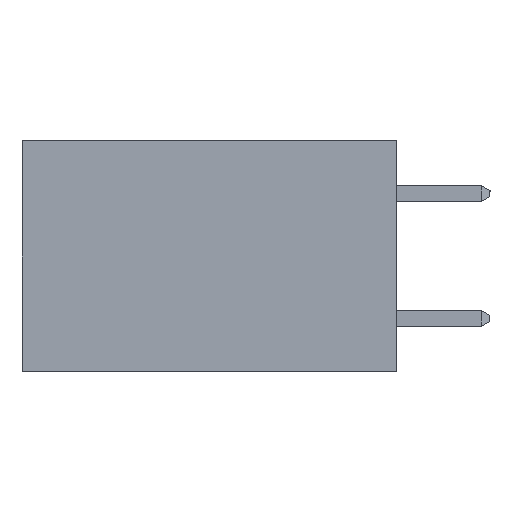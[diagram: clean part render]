
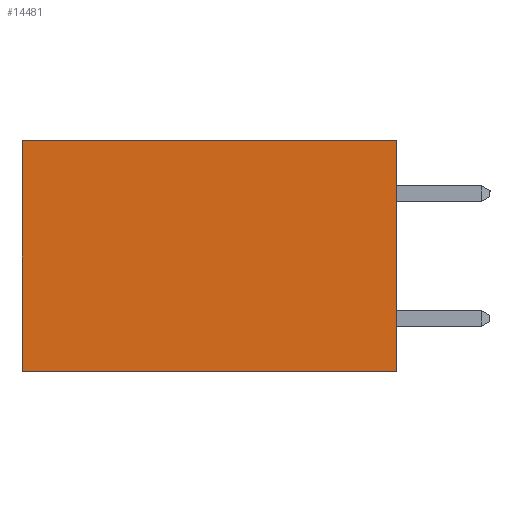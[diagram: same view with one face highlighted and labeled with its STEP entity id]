
A CAD part, left-side view. The second image highlights one B-rep face of the part: STEP entity #14481.
In plain terms, the highlighted planar face has unit normal (-1, 0, 0).
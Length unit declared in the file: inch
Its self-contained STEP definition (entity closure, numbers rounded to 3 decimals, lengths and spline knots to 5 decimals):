
#33 = VECTOR ( 'NONE', #13741, 39.37008 ) ;
#1514 = VECTOR ( 'NONE', #9625, 39.37008 ) ;
#1615 = VERTEX_POINT ( 'NONE', #4444 ) ;
#2081 = DIRECTION ( 'NONE',  ( 1., 0., 0. ) ) ;
#2562 = DIRECTION ( 'NONE',  ( 0., 0., -1. ) ) ;
#2619 = CARTESIAN_POINT ( 'NONE',  ( 0.2615, 0.6, 0. ) ) ;
#3501 = EDGE_CURVE ( 'NONE', #15536, #7044, #13768, .T. ) ;
#4334 = VECTOR ( 'NONE', #6171, 39.37008 ) ;
#4377 = CARTESIAN_POINT ( 'NONE',  ( 0.2615, 0., 0. ) ) ;
#4424 = CARTESIAN_POINT ( 'NONE',  ( 0.2615, 0., -0.37 ) ) ;
#4444 = CARTESIAN_POINT ( 'NONE',  ( 0.2615, 0., -0.37 ) ) ;
#4567 = ORIENTED_EDGE ( 'NONE', *, *, #15018, .F. ) ;
#5959 = LINE ( 'NONE', #11016, #4334 ) ;
#6171 = DIRECTION ( 'NONE',  ( 0., 1., 0. ) ) ;
#7044 = VERTEX_POINT ( 'NONE', #12034 ) ;
#7338 = AXIS2_PLACEMENT_3D ( 'NONE', #16398, #2081, #14927 ) ;
#7967 = ORIENTED_EDGE ( 'NONE', *, *, #3501, .T. ) ;
#8434 = EDGE_CURVE ( 'NONE', #1615, #7044, #5959, .T. ) ;
#9625 = DIRECTION ( 'NONE',  ( 0., 1., 0. ) ) ;
#11016 = CARTESIAN_POINT ( 'NONE',  ( 0.2615, 0., -0.37 ) ) ;
#11141 = ORIENTED_EDGE ( 'NONE', *, *, #14221, .T. ) ;
#11490 = EDGE_LOOP ( 'NONE', ( #7967, #15011, #4567, #11141 ) ) ;
#12034 = CARTESIAN_POINT ( 'NONE',  ( 0.2615, 0.6, -0.37 ) ) ;
#13741 = DIRECTION ( 'NONE',  ( 0., 0., -1. ) ) ;
#13768 = LINE ( 'NONE', #16889, #18731 ) ;
#14221 = EDGE_CURVE ( 'NONE', #18777, #15536, #17357, .T. ) ;
#14481 = ADVANCED_FACE ( 'NONE', ( #19424 ), #17973, .F. ) ;
#14927 = DIRECTION ( 'NONE',  ( 0., 0., -1. ) ) ;
#15011 = ORIENTED_EDGE ( 'NONE', *, *, #8434, .F. ) ;
#15018 = EDGE_CURVE ( 'NONE', #18777, #1615, #20095, .T. ) ;
#15536 = VERTEX_POINT ( 'NONE', #2619 ) ;
#15779 = CARTESIAN_POINT ( 'NONE',  ( 0.2615, 0., 0. ) ) ;
#16398 = CARTESIAN_POINT ( 'NONE',  ( 0.2615, 0., -0.37 ) ) ;
#16889 = CARTESIAN_POINT ( 'NONE',  ( 0.2615, 0.6, -0.37 ) ) ;
#17357 = LINE ( 'NONE', #15779, #1514 ) ;
#17973 = PLANE ( 'NONE',  #7338 ) ;
#18731 = VECTOR ( 'NONE', #2562, 39.37008 ) ;
#18777 = VERTEX_POINT ( 'NONE', #4377 ) ;
#19424 = FACE_OUTER_BOUND ( 'NONE', #11490, .T. ) ;
#20095 = LINE ( 'NONE', #4424, #33 ) ;
